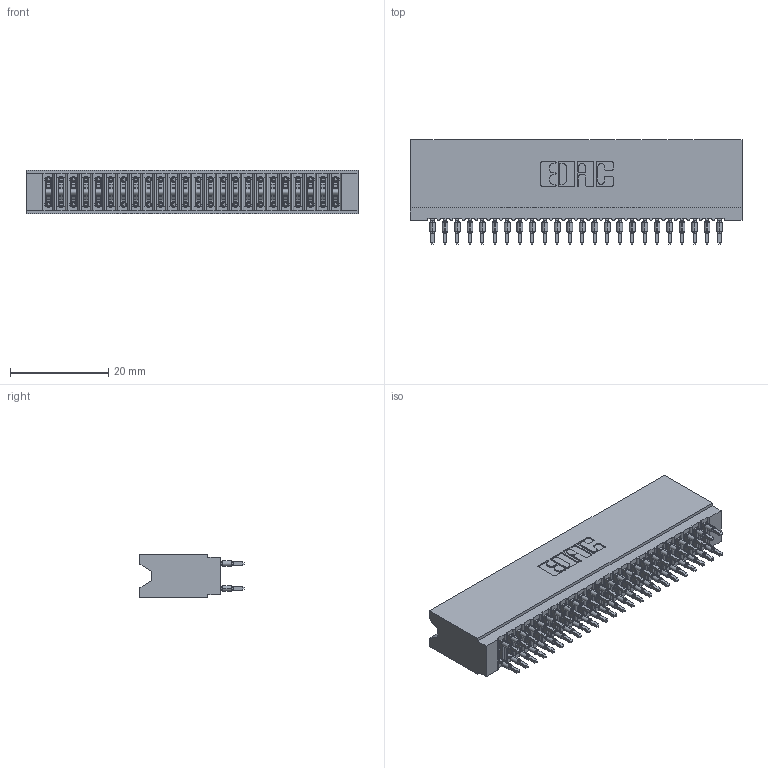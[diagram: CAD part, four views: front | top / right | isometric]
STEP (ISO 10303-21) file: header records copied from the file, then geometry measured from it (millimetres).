
FILE_DESCRIPTION (( 'STEP AP203' ), '1' );
FILE_NAME ('745-048-560-206.STEP', '2026-02-26T18:10:50', ( '' ), ( '' ), 'SwSTEP 2.0', 'SolidWorks 2023', '' );
FILE_SCHEMA (( 'CONFIG_CONTROL_DESIGN' ));
Length unit declared in the file: millimetre
Products named in the file (3): 745-048-560-206; 745-292-001_560; 745 Part_Insulator Option - 06
Assembly tree (49 placements, depth 2):
  745-048-560-206
    745 Part_Insulator Option - 06
    745-292-001_560  x48
Bounding box: 67.56 x 21.22 x 8.89 mm (x, y, z)
Volume: 6348.5 mm3; surface area: 13273.6 mm2
Topology: 49 solids, 49 shells, 4824 faces, 13196 edges, 8380 vertices
Faces by surface type: plane 2504, cylinder 1072, bspline 960, torus 288
Entity records: 43205 total; most frequent: CARTESIAN_POINT 8004, ORIENTED_EDGE 7404, DIRECTION 6488, EDGE_CURVE 3702, LINE 3368, VECTOR 3368, VERTEX_POINT 2364, AXIS2_PLACEMENT_3D 1560
